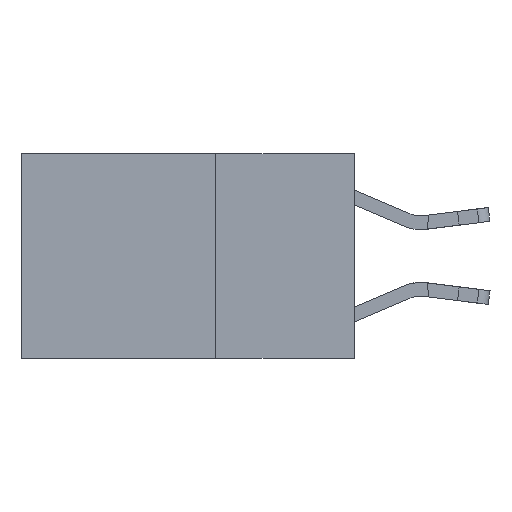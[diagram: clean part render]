
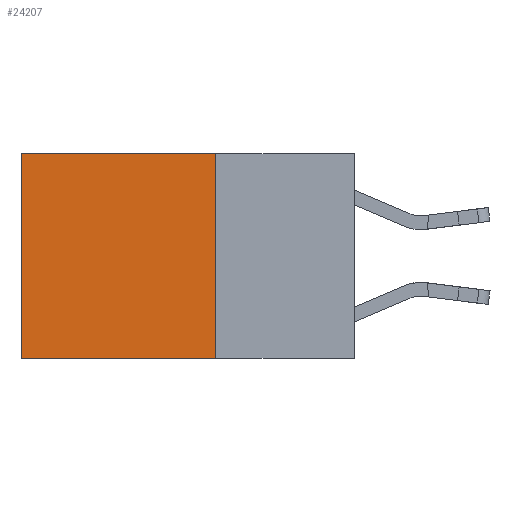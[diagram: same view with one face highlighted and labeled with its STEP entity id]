
A CAD part, left-side view. The second image highlights one B-rep face of the part: STEP entity #24207.
In plain terms, the highlighted planar face has unit normal (-1, 0, 0).
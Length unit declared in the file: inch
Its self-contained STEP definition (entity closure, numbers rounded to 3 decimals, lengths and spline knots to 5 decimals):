
#252 = LINE ( 'NONE', #11951, #22792 ) ;
#789 = DIRECTION ( 'NONE',  ( 0., 1., 0. ) ) ;
#818 = LINE ( 'NONE', #15711, #23368 ) ;
#1346 = DIRECTION ( 'NONE',  ( 0., 0., -1. ) ) ;
#1476 = DIRECTION ( 'NONE',  ( 1., 0., 0. ) ) ;
#1795 = CARTESIAN_POINT ( 'NONE',  ( 0.2625, 0.6, 0. ) ) ;
#1905 = LINE ( 'NONE', #21445, #18147 ) ;
#3653 = ORIENTED_EDGE ( 'NONE', *, *, #15537, .T. ) ;
#5661 = PLANE ( 'NONE',  #10850 ) ;
#7635 = VECTOR ( 'NONE', #26751, 39.37008 ) ;
#10071 = EDGE_CURVE ( 'NONE', #25662, #22941, #1905, .T. ) ;
#10416 = EDGE_CURVE ( 'NONE', #10566, #25662, #252, .T. ) ;
#10566 = VERTEX_POINT ( 'NONE', #14520 ) ;
#10567 = VERTEX_POINT ( 'NONE', #1795 ) ;
#10850 = AXIS2_PLACEMENT_3D ( 'NONE', #14207, #1476, #16316 ) ;
#10966 = DIRECTION ( 'NONE',  ( 0., 1., 0. ) ) ;
#11766 = FACE_OUTER_BOUND ( 'NONE', #22760, .T. ) ;
#11951 = CARTESIAN_POINT ( 'NONE',  ( 0.2625, 0.25, 0. ) ) ;
#13950 = LINE ( 'NONE', #16213, #7635 ) ;
#14207 = CARTESIAN_POINT ( 'NONE',  ( 0.2625, 0.25, 0. ) ) ;
#14520 = CARTESIAN_POINT ( 'NONE',  ( 0.2625, 0.25, 0. ) ) ;
#15537 = EDGE_CURVE ( 'NONE', #10567, #22941, #13950, .T. ) ;
#15711 = CARTESIAN_POINT ( 'NONE',  ( 0.2625, 0.25, 0. ) ) ;
#16213 = CARTESIAN_POINT ( 'NONE',  ( 0.2625, 0.6, 0. ) ) ;
#16316 = DIRECTION ( 'NONE',  ( 0., 0., -1. ) ) ;
#17960 = CARTESIAN_POINT ( 'NONE',  ( 0.2625, 0.25, -0.37 ) ) ;
#18147 = VECTOR ( 'NONE', #10966, 39.37008 ) ;
#19756 = EDGE_CURVE ( 'NONE', #10566, #10567, #818, .T. ) ;
#21445 = CARTESIAN_POINT ( 'NONE',  ( 0.2625, 0.25, -0.37 ) ) ;
#22696 = ORIENTED_EDGE ( 'NONE', *, *, #10071, .F. ) ;
#22760 = EDGE_LOOP ( 'NONE', ( #3653, #22696, #25715, #26615 ) ) ;
#22792 = VECTOR ( 'NONE', #1346, 39.37008 ) ;
#22941 = VERTEX_POINT ( 'NONE', #24989 ) ;
#23368 = VECTOR ( 'NONE', #789, 39.37008 ) ;
#24207 = ADVANCED_FACE ( 'NONE', ( #11766 ), #5661, .F. ) ;
#24989 = CARTESIAN_POINT ( 'NONE',  ( 0.2625, 0.6, -0.37 ) ) ;
#25662 = VERTEX_POINT ( 'NONE', #17960 ) ;
#25715 = ORIENTED_EDGE ( 'NONE', *, *, #10416, .F. ) ;
#26615 = ORIENTED_EDGE ( 'NONE', *, *, #19756, .T. ) ;
#26751 = DIRECTION ( 'NONE',  ( 0., 0., -1. ) ) ;
